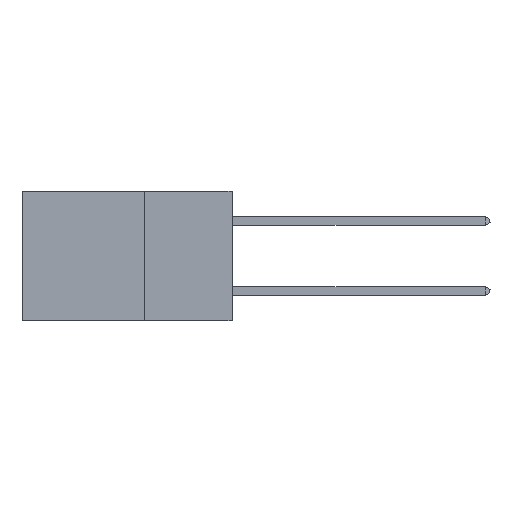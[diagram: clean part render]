
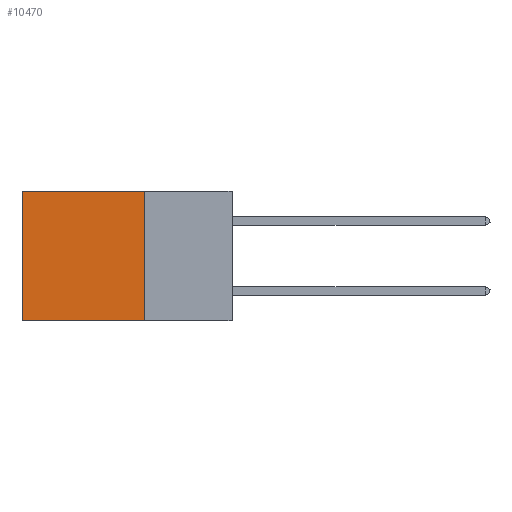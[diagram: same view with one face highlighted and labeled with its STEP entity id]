
A CAD part, left-side view. The second image highlights one B-rep face of the part: STEP entity #10470.
In plain terms, the highlighted planar face has unit normal (-1, 0, 0).
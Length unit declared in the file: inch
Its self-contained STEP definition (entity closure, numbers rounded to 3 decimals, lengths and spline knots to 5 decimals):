
#69 = DIRECTION ( 'NONE',  ( 0., 1., 0. ) ) ;
#123 = CARTESIAN_POINT ( 'NONE',  ( 0.2875, 0.25, 0. ) ) ;
#492 = LINE ( 'NONE', #32282, #22859 ) ;
#681 = DIRECTION ( 'NONE',  ( 0., 0., -1. ) ) ;
#1064 = DIRECTION ( 'NONE',  ( 1., 0., 0. ) ) ;
#4340 = ORIENTED_EDGE ( 'NONE', *, *, #26690, .F. ) ;
#4485 = VERTEX_POINT ( 'NONE', #37691 ) ;
#4838 = FACE_OUTER_BOUND ( 'NONE', #19113, .T. ) ;
#8578 = VECTOR ( 'NONE', #21015, 39.37008 ) ;
#8933 = DIRECTION ( 'NONE',  ( 0., 1., 0. ) ) ;
#10470 = ADVANCED_FACE ( 'NONE', ( #4838 ), #21607, .F. ) ;
#10642 = CARTESIAN_POINT ( 'NONE',  ( 0.2875, 0.25, -0.37 ) ) ;
#11422 = LINE ( 'NONE', #35147, #32019 ) ;
#13875 = EDGE_CURVE ( 'NONE', #24783, #31510, #492, .T. ) ;
#15900 = LINE ( 'NONE', #32776, #8578 ) ;
#19113 = EDGE_LOOP ( 'NONE', ( #24403, #4340, #28232, #19331 ) ) ;
#19331 = ORIENTED_EDGE ( 'NONE', *, *, #13875, .T. ) ;
#19405 = CARTESIAN_POINT ( 'NONE',  ( 0.2875, 0.6, 0. ) ) ;
#19473 = CARTESIAN_POINT ( 'NONE',  ( 0.2875, 0.25, 0. ) ) ;
#21015 = DIRECTION ( 'NONE',  ( 0., 0., -1. ) ) ;
#21607 = PLANE ( 'NONE',  #29500 ) ;
#22859 = VECTOR ( 'NONE', #69, 39.37008 ) ;
#24403 = ORIENTED_EDGE ( 'NONE', *, *, #27988, .T. ) ;
#24783 = VERTEX_POINT ( 'NONE', #19473 ) ;
#24788 = VERTEX_POINT ( 'NONE', #10642 ) ;
#26038 = DIRECTION ( 'NONE',  ( 0., 0., -1. ) ) ;
#26690 = EDGE_CURVE ( 'NONE', #24788, #4485, #11422, .T. ) ;
#26790 = LINE ( 'NONE', #123, #33675 ) ;
#27227 = CARTESIAN_POINT ( 'NONE',  ( 0.2875, 0.25, 0. ) ) ;
#27988 = EDGE_CURVE ( 'NONE', #31510, #4485, #15900, .T. ) ;
#28232 = ORIENTED_EDGE ( 'NONE', *, *, #29068, .F. ) ;
#29068 = EDGE_CURVE ( 'NONE', #24783, #24788, #26790, .T. ) ;
#29500 = AXIS2_PLACEMENT_3D ( 'NONE', #27227, #1064, #681 ) ;
#31510 = VERTEX_POINT ( 'NONE', #19405 ) ;
#32019 = VECTOR ( 'NONE', #8933, 39.37008 ) ;
#32282 = CARTESIAN_POINT ( 'NONE',  ( 0.2875, 0.25, 0. ) ) ;
#32776 = CARTESIAN_POINT ( 'NONE',  ( 0.2875, 0.6, 0. ) ) ;
#33675 = VECTOR ( 'NONE', #26038, 39.37008 ) ;
#35147 = CARTESIAN_POINT ( 'NONE',  ( 0.2875, 0.25, -0.37 ) ) ;
#37691 = CARTESIAN_POINT ( 'NONE',  ( 0.2875, 0.6, -0.37 ) ) ;
